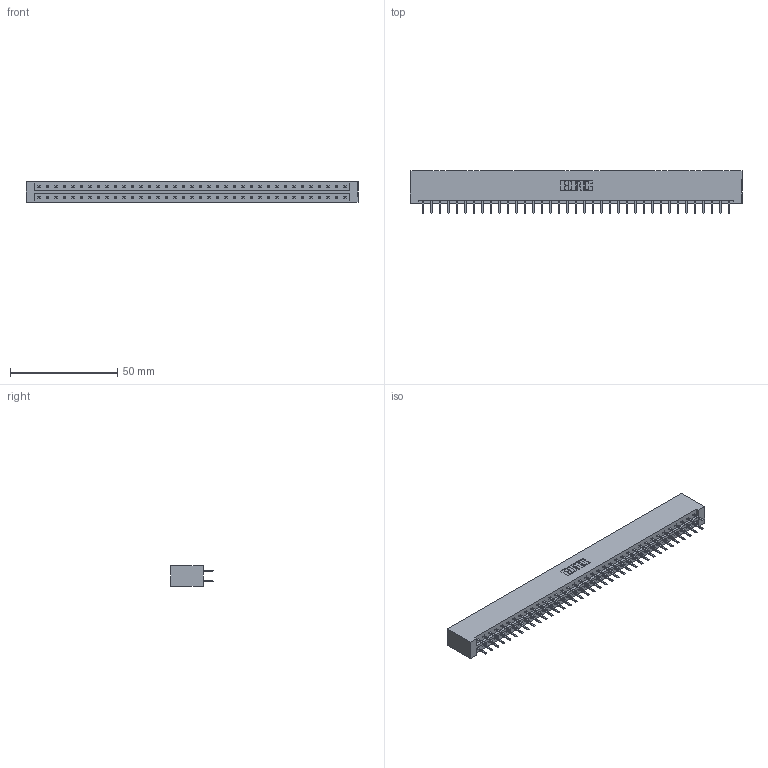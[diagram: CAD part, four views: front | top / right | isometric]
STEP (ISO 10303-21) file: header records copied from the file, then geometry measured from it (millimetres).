
FILE_DESCRIPTION (( 'STEP AP203' ), '1' );
FILE_NAME ('333-074-520-201.STEP', '2018-08-04T21:29:52', ( '' ), ( '' ), 'SwSTEP 2.0', 'SolidWorks 2016', '' );
FILE_SCHEMA (( 'CONFIG_CONTROL_DESIGN' ));
Length unit declared in the file: inch
Products named in the file (3): 333 Part_Lugless; 345-292-001_345-293-120; 333-074-520-201
Assembly tree (75 placements, depth 2):
  333-074-520-201
    333 Part_Lugless
    345-292-001_345-293-120  x74
Bounding box: 154.86 x 20.02 x 9.4 mm (x, y, z)
Volume: 16363.6 mm3; surface area: 19230.4 mm2
Topology: 75 solids, 75 shells, 4250 faces, 12349 edges, 8034 vertices
Faces by surface type: plane 2878, cylinder 1372
Entity records: 24287 total; most frequent: CARTESIAN_POINT 4042, ORIENTED_EDGE 3966, DIRECTION 3443, EDGE_CURVE 1983, VECTOR 1859, LINE 1859, VERTEX_POINT 1318, AXIS2_PLACEMENT_3D 792
